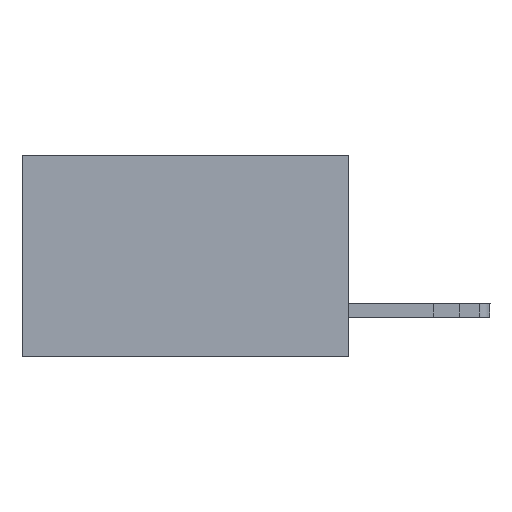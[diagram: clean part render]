
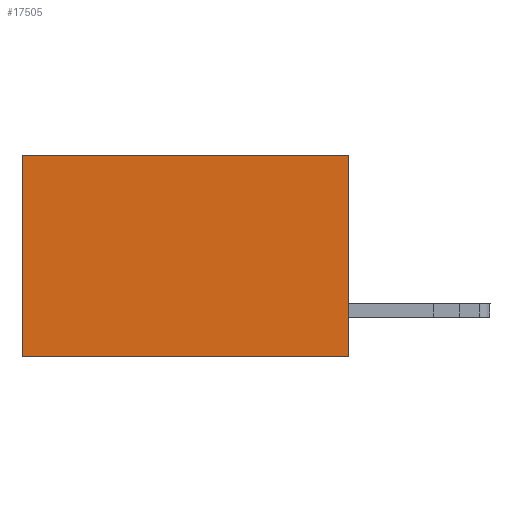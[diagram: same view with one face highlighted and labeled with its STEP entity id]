
A CAD part, left-side view. The second image highlights one B-rep face of the part: STEP entity #17505.
In plain terms, the highlighted planar face has unit normal (-1, 0, 0).
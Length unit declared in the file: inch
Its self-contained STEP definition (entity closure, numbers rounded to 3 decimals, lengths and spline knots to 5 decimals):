
#250 = VECTOR ( 'NONE', #11241, 39.37008 ) ;
#570 = LINE ( 'NONE', #7297, #4489 ) ;
#1351 = CARTESIAN_POINT ( 'NONE',  ( 0.298, 0.6, 0. ) ) ;
#1884 = ORIENTED_EDGE ( 'NONE', *, *, #10820, .T. ) ;
#2219 = CARTESIAN_POINT ( 'NONE',  ( 0.298, 0., 0. ) ) ;
#2822 = CARTESIAN_POINT ( 'NONE',  ( 0.298, 0.6, -0.37 ) ) ;
#3014 = VERTEX_POINT ( 'NONE', #2822 ) ;
#3409 = VECTOR ( 'NONE', #18103, 39.37008 ) ;
#3584 = DIRECTION ( 'NONE',  ( 1., 0., 0. ) ) ;
#4304 = DIRECTION ( 'NONE',  ( 0., 0., -1. ) ) ;
#4489 = VECTOR ( 'NONE', #4304, 39.37008 ) ;
#4639 = LINE ( 'NONE', #9836, #17637 ) ;
#4859 = EDGE_CURVE ( 'NONE', #9261, #3014, #4639, .T. ) ;
#5635 = CARTESIAN_POINT ( 'NONE',  ( 0.298, 0., -0.37 ) ) ;
#5781 = LINE ( 'NONE', #7920, #250 ) ;
#7297 = CARTESIAN_POINT ( 'NONE',  ( 0.298, 0.6, 0. ) ) ;
#7920 = CARTESIAN_POINT ( 'NONE',  ( 0.298, 0., 0. ) ) ;
#8192 = ORIENTED_EDGE ( 'NONE', *, *, #11306, .F. ) ;
#9261 = VERTEX_POINT ( 'NONE', #5635 ) ;
#9730 = VERTEX_POINT ( 'NONE', #1351 ) ;
#9836 = CARTESIAN_POINT ( 'NONE',  ( 0.298, 0., -0.37 ) ) ;
#10348 = ORIENTED_EDGE ( 'NONE', *, *, #16604, .T. ) ;
#10820 = EDGE_CURVE ( 'NONE', #17879, #9730, #5781, .T. ) ;
#11240 = PLANE ( 'NONE',  #18328 ) ;
#11241 = DIRECTION ( 'NONE',  ( 0., 1., 0. ) ) ;
#11306 = EDGE_CURVE ( 'NONE', #17879, #9261, #17375, .T. ) ;
#11994 = CARTESIAN_POINT ( 'NONE',  ( 0.298, 0., 0. ) ) ;
#12702 = DIRECTION ( 'NONE',  ( 0., 0., -1. ) ) ;
#14314 = DIRECTION ( 'NONE',  ( 0., 1., 0. ) ) ;
#16364 = CARTESIAN_POINT ( 'NONE',  ( 0.298, 0., 0. ) ) ;
#16604 = EDGE_CURVE ( 'NONE', #9730, #3014, #570, .T. ) ;
#16906 = ORIENTED_EDGE ( 'NONE', *, *, #4859, .F. ) ;
#17375 = LINE ( 'NONE', #16364, #3409 ) ;
#17505 = ADVANCED_FACE ( 'NONE', ( #18193 ), #11240, .F. ) ;
#17637 = VECTOR ( 'NONE', #14314, 39.37008 ) ;
#17879 = VERTEX_POINT ( 'NONE', #11994 ) ;
#18103 = DIRECTION ( 'NONE',  ( 0., 0., -1. ) ) ;
#18193 = FACE_OUTER_BOUND ( 'NONE', #18374, .T. ) ;
#18328 = AXIS2_PLACEMENT_3D ( 'NONE', #2219, #3584, #12702 ) ;
#18374 = EDGE_LOOP ( 'NONE', ( #10348, #16906, #8192, #1884 ) ) ;
